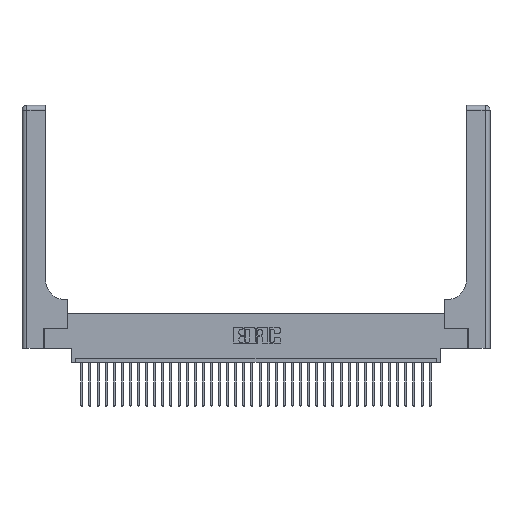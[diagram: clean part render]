
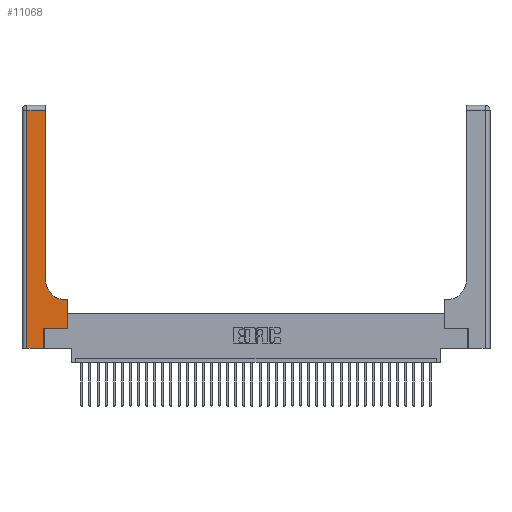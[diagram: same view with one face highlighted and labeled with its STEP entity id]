
A CAD part, top view. The second image highlights one B-rep face of the part: STEP entity #11068.
In plain terms, the highlighted planar face has unit normal (0, 0, 1).
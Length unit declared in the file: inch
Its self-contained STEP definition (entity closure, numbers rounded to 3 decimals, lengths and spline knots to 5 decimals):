
#835 = CARTESIAN_POINT ( 'NONE',  ( 0.5585, 0.6, 0.37 ) ) ;
#955 = ORIENTED_EDGE ( 'NONE', *, *, #4862, .T. ) ;
#964 = DIRECTION ( 'NONE',  ( 0., -1., 0. ) ) ;
#1400 = VERTEX_POINT ( 'NONE', #17843 ) ;
#1656 = ORIENTED_EDGE ( 'NONE', *, *, #34618, .T. ) ;
#1994 = DIRECTION ( 'NONE',  ( -1., 0., 0. ) ) ;
#2014 = CIRCLE ( 'NONE', #20672, 0.25 ) ;
#2692 = LINE ( 'NONE', #30222, #35892 ) ;
#2918 = LINE ( 'NONE', #23935, #20863 ) ;
#3565 = CARTESIAN_POINT ( 'NONE',  ( 0.2915, 0.6, 0.37 ) ) ;
#4140 = VECTOR ( 'NONE', #38064, 39.37008 ) ;
#4226 = ORIENTED_EDGE ( 'NONE', *, *, #32835, .T. ) ;
#4336 = LINE ( 'NONE', #30432, #36649 ) ;
#4862 = EDGE_CURVE ( 'NONE', #28261, #27638, #28167, .T. ) ;
#4937 = ORIENTED_EDGE ( 'NONE', *, *, #14826, .T. ) ;
#5562 = CARTESIAN_POINT ( 'NONE',  ( 0.5415, 0.85, 0.37 ) ) ;
#5708 = VECTOR ( 'NONE', #9108, 39.37008 ) ;
#6157 = LINE ( 'NONE', #35532, #5708 ) ;
#7258 = ORIENTED_EDGE ( 'NONE', *, *, #24837, .T. ) ;
#7295 = EDGE_CURVE ( 'NONE', #27352, #30274, #2692, .T. ) ;
#8130 = DIRECTION ( 'NONE',  ( 0., 0., -1. ) ) ;
#8184 = VERTEX_POINT ( 'NONE', #32394 ) ;
#9106 = EDGE_LOOP ( 'NONE', ( #4937, #4226, #11630, #7258, #1656, #19158, #33414, #955, #23032 ) ) ;
#9108 = DIRECTION ( 'NONE',  ( 0., 1., 0. ) ) ;
#9488 = VECTOR ( 'NONE', #1994, 39.37008 ) ;
#9870 = VERTEX_POINT ( 'NONE', #31016 ) ;
#11068 = ADVANCED_FACE ( 'NONE', ( #31342 ), #16909, .F. ) ;
#11630 = ORIENTED_EDGE ( 'NONE', *, *, #7295, .T. ) ;
#12297 = VERTEX_POINT ( 'NONE', #26851 ) ;
#14826 = EDGE_CURVE ( 'NONE', #12297, #16570, #6157, .T. ) ;
#14865 = DIRECTION ( 'NONE',  ( 1., 0., 0. ) ) ;
#15776 = CARTESIAN_POINT ( 'NONE',  ( 0., 0., 0.37 ) ) ;
#16041 = AXIS2_PLACEMENT_3D ( 'NONE', #22708, #8130, #28494 ) ;
#16570 = VERTEX_POINT ( 'NONE', #21041 ) ;
#16782 = CARTESIAN_POINT ( 'NONE',  ( 0.06, 0., 0.37 ) ) ;
#16909 = PLANE ( 'NONE',  #16041 ) ;
#17843 = CARTESIAN_POINT ( 'NONE',  ( 0.5585, 0.25, 0.37 ) ) ;
#18328 = EDGE_CURVE ( 'NONE', #9870, #1400, #22124, .T. ) ;
#18706 = DIRECTION ( 'NONE',  ( 0., 1., 0. ) ) ;
#18723 = DIRECTION ( 'NONE',  ( 1., 0., 0. ) ) ;
#19158 = ORIENTED_EDGE ( 'NONE', *, *, #18328, .T. ) ;
#20243 = DIRECTION ( 'NONE',  ( 0., 0., -1. ) ) ;
#20613 = CARTESIAN_POINT ( 'NONE',  ( 0.5415, 0.6, 0.37 ) ) ;
#20672 = AXIS2_PLACEMENT_3D ( 'NONE', #5562, #20243, #14865 ) ;
#20863 = VECTOR ( 'NONE', #24188, 39.37008 ) ;
#20904 = CARTESIAN_POINT ( 'NONE',  ( 0.269, 0.25, 0.37 ) ) ;
#21041 = CARTESIAN_POINT ( 'NONE',  ( 0.2915, 2.94, 0.37 ) ) ;
#21286 = CARTESIAN_POINT ( 'NONE',  ( 0.06, 2.94, 0.37 ) ) ;
#21354 = DIRECTION ( 'NONE',  ( -1., 0., 0. ) ) ;
#21665 = EDGE_CURVE ( 'NONE', #27638, #12297, #2014, .T. ) ;
#22124 = LINE ( 'NONE', #20904, #4140 ) ;
#22708 = CARTESIAN_POINT ( 'NONE',  ( 0., 3., 0.37 ) ) ;
#23032 = ORIENTED_EDGE ( 'NONE', *, *, #21665, .T. ) ;
#23935 = CARTESIAN_POINT ( 'NONE',  ( 0.5585, 0.25, 0.37 ) ) ;
#24188 = DIRECTION ( 'NONE',  ( 0., 1., 0. ) ) ;
#24837 = EDGE_CURVE ( 'NONE', #30274, #8184, #29794, .T. ) ;
#26623 = EDGE_CURVE ( 'NONE', #1400, #28261, #2918, .T. ) ;
#26851 = CARTESIAN_POINT ( 'NONE',  ( 0.2915, 0.85, 0.37 ) ) ;
#27352 = VERTEX_POINT ( 'NONE', #21286 ) ;
#27638 = VERTEX_POINT ( 'NONE', #20613 ) ;
#27919 = VECTOR ( 'NONE', #18723, 39.37008 ) ;
#28167 = LINE ( 'NONE', #3565, #35139 ) ;
#28261 = VERTEX_POINT ( 'NONE', #835 ) ;
#28494 = DIRECTION ( 'NONE',  ( -1., 0., 0. ) ) ;
#28776 = CARTESIAN_POINT ( 'NONE',  ( 0., 2.94, 0.37 ) ) ;
#29794 = LINE ( 'NONE', #15776, #27919 ) ;
#30222 = CARTESIAN_POINT ( 'NONE',  ( 0.06, 3., 0.37 ) ) ;
#30274 = VERTEX_POINT ( 'NONE', #16782 ) ;
#30432 = CARTESIAN_POINT ( 'NONE',  ( 0.269, 0., 0.37 ) ) ;
#31016 = CARTESIAN_POINT ( 'NONE',  ( 0.269, 0.25, 0.37 ) ) ;
#31342 = FACE_OUTER_BOUND ( 'NONE', #9106, .T. ) ;
#32394 = CARTESIAN_POINT ( 'NONE',  ( 0.269, 0., 0.37 ) ) ;
#32835 = EDGE_CURVE ( 'NONE', #16570, #27352, #37623, .T. ) ;
#33414 = ORIENTED_EDGE ( 'NONE', *, *, #26623, .T. ) ;
#34618 = EDGE_CURVE ( 'NONE', #8184, #9870, #4336, .T. ) ;
#35139 = VECTOR ( 'NONE', #21354, 39.37008 ) ;
#35532 = CARTESIAN_POINT ( 'NONE',  ( 0.2915, 3., 0.37 ) ) ;
#35892 = VECTOR ( 'NONE', #964, 39.37008 ) ;
#36649 = VECTOR ( 'NONE', #18706, 39.37008 ) ;
#37623 = LINE ( 'NONE', #28776, #9488 ) ;
#38064 = DIRECTION ( 'NONE',  ( 1., 0., 0. ) ) ;
